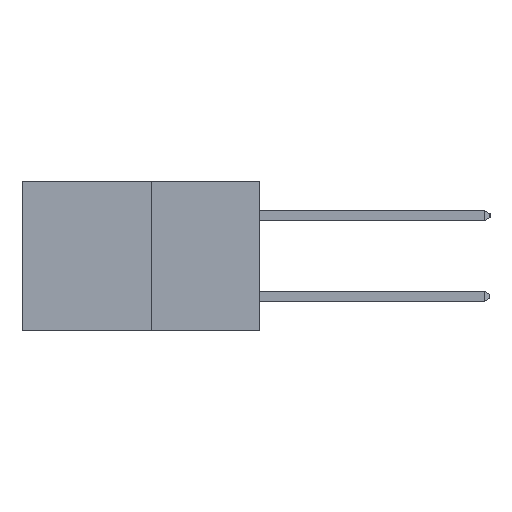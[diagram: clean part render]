
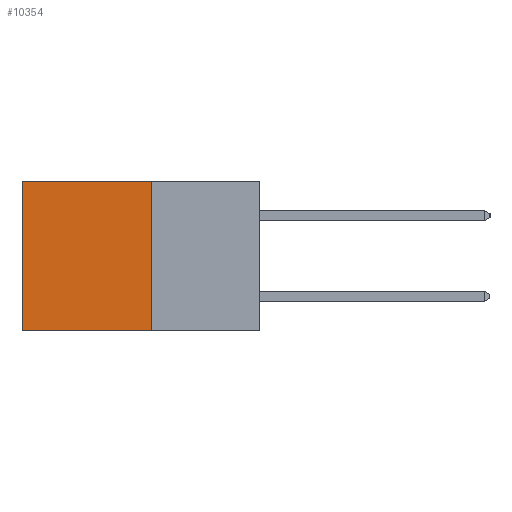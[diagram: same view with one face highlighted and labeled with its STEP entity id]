
A CAD part, left-side view. The second image highlights one B-rep face of the part: STEP entity #10354.
In plain terms, the highlighted planar face has unit normal (-1, 0, 0).
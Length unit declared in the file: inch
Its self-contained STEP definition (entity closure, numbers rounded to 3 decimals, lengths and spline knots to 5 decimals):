
#83 = VECTOR ( 'NONE', #7181, 39.37008 ) ;
#148 = ORIENTED_EDGE ( 'NONE', *, *, #2911, .T. ) ;
#286 = DIRECTION ( 'NONE',  ( 0., 1., 0. ) ) ;
#438 = CARTESIAN_POINT ( 'NONE',  ( 0.277, 0.27, 0. ) ) ;
#1096 = CARTESIAN_POINT ( 'NONE',  ( 0.277, 0.59, -0.37 ) ) ;
#1420 = VERTEX_POINT ( 'NONE', #9724 ) ;
#1642 = VERTEX_POINT ( 'NONE', #8151 ) ;
#2158 = LINE ( 'NONE', #1096, #83 ) ;
#2214 = ORIENTED_EDGE ( 'NONE', *, *, #5798, .F. ) ;
#2911 = EDGE_CURVE ( 'NONE', #10204, #1420, #7749, .T. ) ;
#3000 = CARTESIAN_POINT ( 'NONE',  ( 0.277, 0.27, -0.37 ) ) ;
#3994 = CARTESIAN_POINT ( 'NONE',  ( 0.277, 0.27, 0. ) ) ;
#4056 = LINE ( 'NONE', #3000, #10311 ) ;
#4304 = DIRECTION ( 'NONE',  ( 0., 0., -1. ) ) ;
#5184 = AXIS2_PLACEMENT_3D ( 'NONE', #5922, #10132, #7636 ) ;
#5798 = EDGE_CURVE ( 'NONE', #10204, #1642, #4056, .T. ) ;
#5865 = VECTOR ( 'NONE', #9356, 39.37008 ) ;
#5922 = CARTESIAN_POINT ( 'NONE',  ( 0.277, 0.27, -0.37 ) ) ;
#6039 = ORIENTED_EDGE ( 'NONE', *, *, #9280, .T. ) ;
#6785 = PLANE ( 'NONE',  #5184 ) ;
#6938 = VERTEX_POINT ( 'NONE', #10559 ) ;
#7075 = EDGE_CURVE ( 'NONE', #1642, #6938, #8384, .T. ) ;
#7181 = DIRECTION ( 'NONE',  ( 0., 0., -1. ) ) ;
#7485 = VECTOR ( 'NONE', #286, 39.37008 ) ;
#7636 = DIRECTION ( 'NONE',  ( 0., 0., -1. ) ) ;
#7681 = FACE_OUTER_BOUND ( 'NONE', #9179, .T. ) ;
#7749 = LINE ( 'NONE', #438, #7485 ) ;
#8151 = CARTESIAN_POINT ( 'NONE',  ( 0.277, 0.27, -0.37 ) ) ;
#8384 = LINE ( 'NONE', #9400, #5865 ) ;
#8802 = ORIENTED_EDGE ( 'NONE', *, *, #7075, .F. ) ;
#9179 = EDGE_LOOP ( 'NONE', ( #6039, #8802, #2214, #148 ) ) ;
#9280 = EDGE_CURVE ( 'NONE', #1420, #6938, #2158, .T. ) ;
#9356 = DIRECTION ( 'NONE',  ( 0., 1., 0. ) ) ;
#9400 = CARTESIAN_POINT ( 'NONE',  ( 0.277, 0.27, -0.37 ) ) ;
#9724 = CARTESIAN_POINT ( 'NONE',  ( 0.277, 0.59, 0. ) ) ;
#10132 = DIRECTION ( 'NONE',  ( 1., 0., 0. ) ) ;
#10204 = VERTEX_POINT ( 'NONE', #3994 ) ;
#10311 = VECTOR ( 'NONE', #4304, 39.37008 ) ;
#10354 = ADVANCED_FACE ( 'NONE', ( #7681 ), #6785, .F. ) ;
#10559 = CARTESIAN_POINT ( 'NONE',  ( 0.277, 0.59, -0.37 ) ) ;
